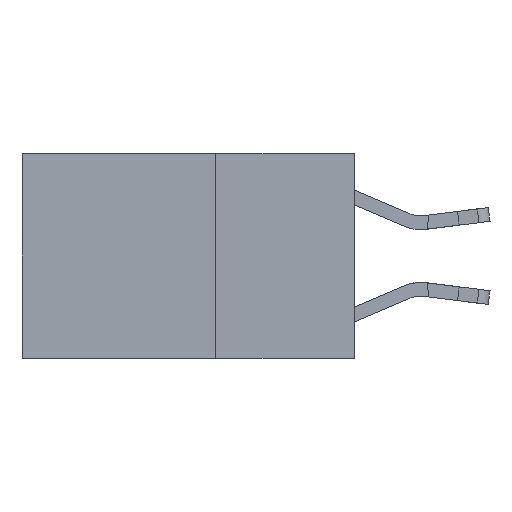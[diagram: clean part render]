
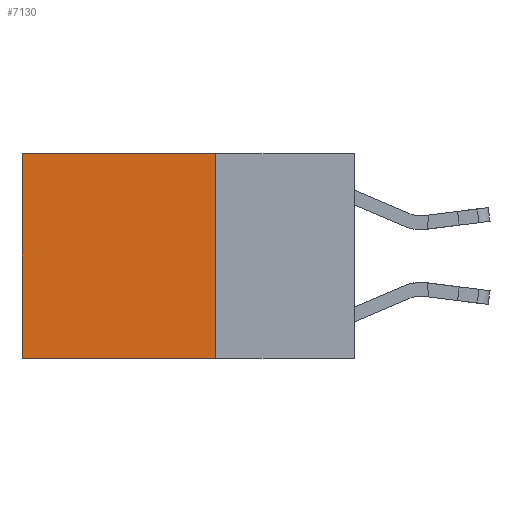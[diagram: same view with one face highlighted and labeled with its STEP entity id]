
A CAD part, left-side view. The second image highlights one B-rep face of the part: STEP entity #7130.
In plain terms, the highlighted planar face has unit normal (-1, 0, 0).
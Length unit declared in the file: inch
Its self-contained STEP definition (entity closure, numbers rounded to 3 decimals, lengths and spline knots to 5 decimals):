
#612 = EDGE_CURVE ( 'NONE', #6824, #15573, #2170, .T. ) ;
#1467 = VECTOR ( 'NONE', #15515, 39.37008 ) ;
#2170 = LINE ( 'NONE', #17669, #8501 ) ;
#3010 = DIRECTION ( 'NONE',  ( 1., 0., 0. ) ) ;
#3071 = CARTESIAN_POINT ( 'NONE',  ( 0.2625, 0.25, 0. ) ) ;
#3902 = EDGE_CURVE ( 'NONE', #15573, #15127, #11605, .T. ) ;
#5274 = EDGE_LOOP ( 'NONE', ( #17096, #11327, #16562, #21492 ) ) ;
#5769 = CARTESIAN_POINT ( 'NONE',  ( 0.2625, 0.25, -0.37 ) ) ;
#6824 = VERTEX_POINT ( 'NONE', #7598 ) ;
#7130 = ADVANCED_FACE ( 'NONE', ( #10634 ), #18239, .F. ) ;
#7598 = CARTESIAN_POINT ( 'NONE',  ( 0.2625, 0.25, 0. ) ) ;
#7655 = CARTESIAN_POINT ( 'NONE',  ( 0.2625, 0.25, -0.37 ) ) ;
#8236 = VERTEX_POINT ( 'NONE', #11685 ) ;
#8501 = VECTOR ( 'NONE', #15892, 39.37008 ) ;
#10634 = FACE_OUTER_BOUND ( 'NONE', #5274, .T. ) ;
#11206 = LINE ( 'NONE', #16518, #15012 ) ;
#11327 = ORIENTED_EDGE ( 'NONE', *, *, #3902, .F. ) ;
#11523 = CARTESIAN_POINT ( 'NONE',  ( 0.2625, 0.6, -0.37 ) ) ;
#11605 = LINE ( 'NONE', #7655, #1467 ) ;
#11685 = CARTESIAN_POINT ( 'NONE',  ( 0.2625, 0.6, 0. ) ) ;
#13963 = EDGE_CURVE ( 'NONE', #8236, #15127, #11206, .T. ) ;
#14814 = VECTOR ( 'NONE', #18545, 39.37008 ) ;
#15012 = VECTOR ( 'NONE', #18552, 39.37008 ) ;
#15127 = VERTEX_POINT ( 'NONE', #11523 ) ;
#15515 = DIRECTION ( 'NONE',  ( 0., 1., 0. ) ) ;
#15573 = VERTEX_POINT ( 'NONE', #5769 ) ;
#15892 = DIRECTION ( 'NONE',  ( 0., 0., -1. ) ) ;
#16518 = CARTESIAN_POINT ( 'NONE',  ( 0.2625, 0.6, 0. ) ) ;
#16562 = ORIENTED_EDGE ( 'NONE', *, *, #612, .F. ) ;
#17096 = ORIENTED_EDGE ( 'NONE', *, *, #13963, .T. ) ;
#17669 = CARTESIAN_POINT ( 'NONE',  ( 0.2625, 0.25, 0. ) ) ;
#18239 = PLANE ( 'NONE',  #23804 ) ;
#18362 = CARTESIAN_POINT ( 'NONE',  ( 0.2625, 0.25, 0. ) ) ;
#18545 = DIRECTION ( 'NONE',  ( 0., 1., 0. ) ) ;
#18552 = DIRECTION ( 'NONE',  ( 0., 0., -1. ) ) ;
#20059 = LINE ( 'NONE', #3071, #14814 ) ;
#21492 = ORIENTED_EDGE ( 'NONE', *, *, #22081, .T. ) ;
#21943 = DIRECTION ( 'NONE',  ( 0., 0., -1. ) ) ;
#22081 = EDGE_CURVE ( 'NONE', #6824, #8236, #20059, .T. ) ;
#23804 = AXIS2_PLACEMENT_3D ( 'NONE', #18362, #3010, #21943 ) ;
